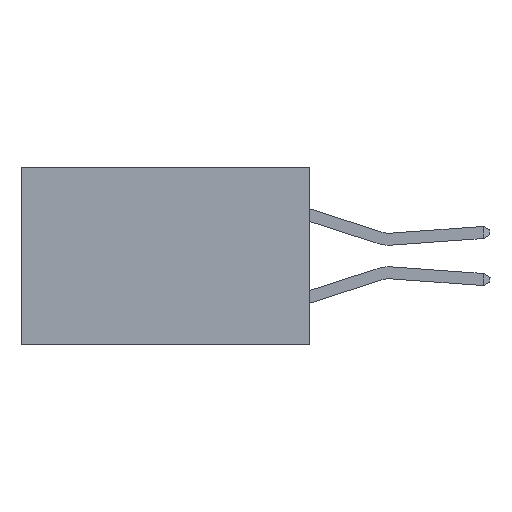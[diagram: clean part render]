
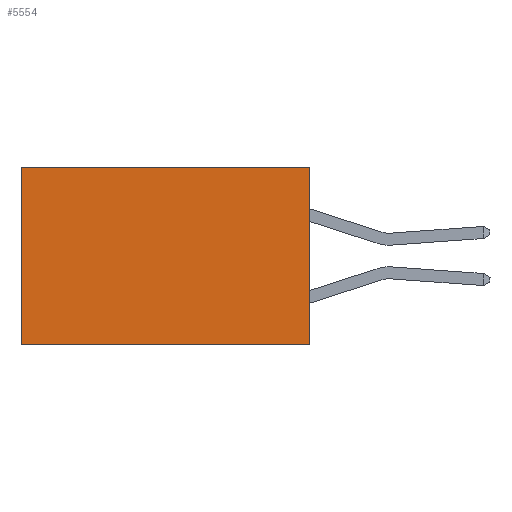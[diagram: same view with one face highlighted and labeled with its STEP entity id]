
A CAD part, left-side view. The second image highlights one B-rep face of the part: STEP entity #5554.
In plain terms, the highlighted planar face has unit normal (-1, 0, 0).
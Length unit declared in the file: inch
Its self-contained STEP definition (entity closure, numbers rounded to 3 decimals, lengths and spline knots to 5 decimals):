
#834 = CARTESIAN_POINT ( 'NONE',  ( 0.298, 0., -0.37 ) ) ;
#1238 = VERTEX_POINT ( 'NONE', #4671 ) ;
#1466 = PLANE ( 'NONE',  #3975 ) ;
#2268 = DIRECTION ( 'NONE',  ( 0., 1., 0. ) ) ;
#3276 = DIRECTION ( 'NONE',  ( 0., 0., -1. ) ) ;
#3330 = EDGE_CURVE ( 'NONE', #19827, #8823, #19072, .T. ) ;
#3504 = CARTESIAN_POINT ( 'NONE',  ( 0.298, 0., 0. ) ) ;
#3890 = VERTEX_POINT ( 'NONE', #13887 ) ;
#3975 = AXIS2_PLACEMENT_3D ( 'NONE', #17745, #18594, #7057 ) ;
#4148 = EDGE_CURVE ( 'NONE', #3890, #19827, #15458, .T. ) ;
#4354 = LINE ( 'NONE', #3504, #14064 ) ;
#4671 = CARTESIAN_POINT ( 'NONE',  ( 0.298, 0.6, 0. ) ) ;
#4861 = EDGE_LOOP ( 'NONE', ( #5944, #22070, #12359, #18240 ) ) ;
#5440 = CARTESIAN_POINT ( 'NONE',  ( 0.298, 0.6, -0.37 ) ) ;
#5554 = ADVANCED_FACE ( 'NONE', ( #21621 ), #1466, .F. ) ;
#5944 = ORIENTED_EDGE ( 'NONE', *, *, #13650, .T. ) ;
#7057 = DIRECTION ( 'NONE',  ( 0., 0., -1. ) ) ;
#7873 = CARTESIAN_POINT ( 'NONE',  ( 0.298, 0., -0.37 ) ) ;
#8823 = VERTEX_POINT ( 'NONE', #5440 ) ;
#10040 = DIRECTION ( 'NONE',  ( 0., 0., -1. ) ) ;
#12359 = ORIENTED_EDGE ( 'NONE', *, *, #4148, .F. ) ;
#13650 = EDGE_CURVE ( 'NONE', #1238, #8823, #21070, .T. ) ;
#13887 = CARTESIAN_POINT ( 'NONE',  ( 0.298, 0., 0. ) ) ;
#14064 = VECTOR ( 'NONE', #16274, 39.37008 ) ;
#14350 = VECTOR ( 'NONE', #2268, 39.37008 ) ;
#15458 = LINE ( 'NONE', #21770, #19587 ) ;
#16274 = DIRECTION ( 'NONE',  ( 0., 1., 0. ) ) ;
#16954 = VECTOR ( 'NONE', #10040, 39.37008 ) ;
#17745 = CARTESIAN_POINT ( 'NONE',  ( 0.298, 0., 0. ) ) ;
#18240 = ORIENTED_EDGE ( 'NONE', *, *, #20001, .T. ) ;
#18594 = DIRECTION ( 'NONE',  ( 1., 0., 0. ) ) ;
#19072 = LINE ( 'NONE', #7873, #14350 ) ;
#19587 = VECTOR ( 'NONE', #3276, 39.37008 ) ;
#19827 = VERTEX_POINT ( 'NONE', #834 ) ;
#20001 = EDGE_CURVE ( 'NONE', #3890, #1238, #4354, .T. ) ;
#20777 = CARTESIAN_POINT ( 'NONE',  ( 0.298, 0.6, 0. ) ) ;
#21070 = LINE ( 'NONE', #20777, #16954 ) ;
#21621 = FACE_OUTER_BOUND ( 'NONE', #4861, .T. ) ;
#21770 = CARTESIAN_POINT ( 'NONE',  ( 0.298, 0., 0. ) ) ;
#22070 = ORIENTED_EDGE ( 'NONE', *, *, #3330, .F. ) ;
